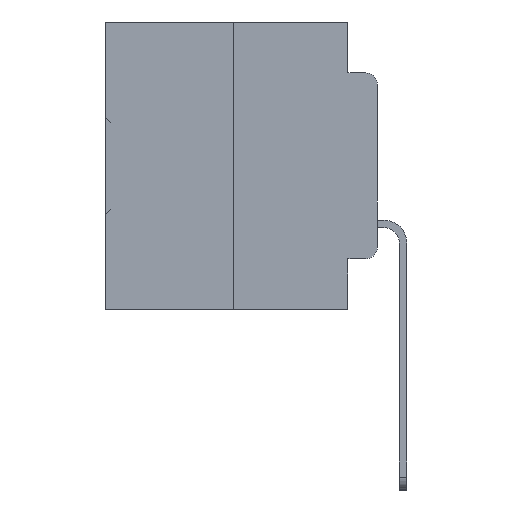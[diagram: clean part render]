
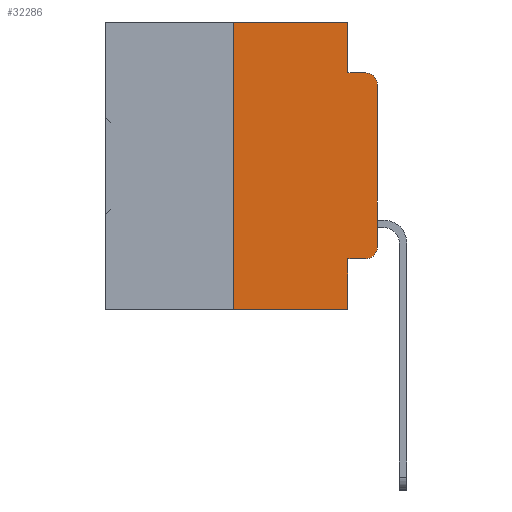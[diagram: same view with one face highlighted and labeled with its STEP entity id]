
A CAD part, left-side view. The second image highlights one B-rep face of the part: STEP entity #32286.
In plain terms, the highlighted planar face has unit normal (-1, 0, 0).
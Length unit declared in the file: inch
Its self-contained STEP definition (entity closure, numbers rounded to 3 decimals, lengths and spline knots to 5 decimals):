
#32 = EDGE_CURVE ( 'NONE', #3070, #14172, #7735, .T. ) ;
#1850 = DIRECTION ( 'NONE',  ( 0., 0., -1. ) ) ;
#1936 = VERTEX_POINT ( 'NONE', #9172 ) ;
#2328 = EDGE_CURVE ( 'NONE', #14172, #29148, #20751, .T. ) ;
#2523 = ORIENTED_EDGE ( 'NONE', *, *, #2328, .T. ) ;
#2650 = ORIENTED_EDGE ( 'NONE', *, *, #19686, .T. ) ;
#3070 = VERTEX_POINT ( 'NONE', #14114 ) ;
#3313 = ORIENTED_EDGE ( 'NONE', *, *, #5236, .F. ) ;
#3793 = CIRCLE ( 'NONE', #24096, 0.02 ) ;
#3899 = ORIENTED_EDGE ( 'NONE', *, *, #9823, .F. ) ;
#4029 = CARTESIAN_POINT ( 'NONE',  ( 0., 0.051, -0.0885 ) ) ;
#4086 = ORIENTED_EDGE ( 'NONE', *, *, #6081, .F. ) ;
#4285 = ORIENTED_EDGE ( 'NONE', *, *, #34201, .F. ) ;
#5115 = CARTESIAN_POINT ( 'NONE',  ( 0., 0.051, 0. ) ) ;
#5236 = EDGE_CURVE ( 'NONE', #16485, #1936, #21415, .T. ) ;
#5287 = ORIENTED_EDGE ( 'NONE', *, *, #8079, .T. ) ;
#5360 = ORIENTED_EDGE ( 'NONE', *, *, #6774, .F. ) ;
#5570 = CARTESIAN_POINT ( 'NONE',  ( 0., 0.25, 0. ) ) ;
#5973 = CARTESIAN_POINT ( 'NONE',  ( 0., 0.051, -0.0885 ) ) ;
#6081 = EDGE_CURVE ( 'NONE', #24636, #24177, #11952, .T. ) ;
#6456 = CARTESIAN_POINT ( 'NONE',  ( 0., 0.473, -0.5 ) ) ;
#6774 = EDGE_CURVE ( 'NONE', #10427, #34752, #24679, .T. ) ;
#6993 = ORIENTED_EDGE ( 'NONE', *, *, #25337, .T. ) ;
#7388 = PLANE ( 'NONE',  #17544 ) ;
#7418 = ORIENTED_EDGE ( 'NONE', *, *, #32, .T. ) ;
#7715 = VECTOR ( 'NONE', #22508, 39.37008 ) ;
#7735 = CIRCLE ( 'NONE', #28140, 0.02 ) ;
#8079 = EDGE_CURVE ( 'NONE', #11602, #34752, #12018, .T. ) ;
#9172 = CARTESIAN_POINT ( 'NONE',  ( 0., 0.02, -0.0885 ) ) ;
#9292 = VECTOR ( 'NONE', #30020, 39.37008 ) ;
#9823 = EDGE_CURVE ( 'NONE', #24177, #16485, #28070, .T. ) ;
#10196 = DIRECTION ( 'NONE',  ( 1., 0., 0. ) ) ;
#10427 = VERTEX_POINT ( 'NONE', #29548 ) ;
#11602 = VERTEX_POINT ( 'NONE', #20110 ) ;
#11652 = DIRECTION ( 'NONE',  ( 0., 0., 1. ) ) ;
#11952 = LINE ( 'NONE', #12339, #25570 ) ;
#12018 = LINE ( 'NONE', #6456, #20133 ) ;
#12339 = CARTESIAN_POINT ( 'NONE',  ( 0., 0.473, 0. ) ) ;
#12803 = CARTESIAN_POINT ( 'NONE',  ( 0., 0.051, -0.4115 ) ) ;
#13549 = VECTOR ( 'NONE', #11652, 39.37008 ) ;
#14114 = CARTESIAN_POINT ( 'NONE',  ( 0., 0.02, -0.4115 ) ) ;
#14172 = VERTEX_POINT ( 'NONE', #30657 ) ;
#15082 = DIRECTION ( 'NONE',  ( 0., -1., 0. ) ) ;
#15665 = DIRECTION ( 'NONE',  ( 0., -1., 0. ) ) ;
#16280 = DIRECTION ( 'NONE',  ( 0., 0., -1. ) ) ;
#16485 = VERTEX_POINT ( 'NONE', #4029 ) ;
#17544 = AXIS2_PLACEMENT_3D ( 'NONE', #18353, #10196, #29260 ) ;
#18353 = CARTESIAN_POINT ( 'NONE',  ( 0., 0.473, 0. ) ) ;
#18394 = FACE_OUTER_BOUND ( 'NONE', #20306, .T. ) ;
#18772 = CARTESIAN_POINT ( 'NONE',  ( 0., 0.25, 0. ) ) ;
#18903 = DIRECTION ( 'NONE',  ( -1., 0., 0. ) ) ;
#19545 = DIRECTION ( 'NONE',  ( 0., 0., 1. ) ) ;
#19686 = EDGE_CURVE ( 'NONE', #29148, #1936, #3793, .T. ) ;
#20110 = CARTESIAN_POINT ( 'NONE',  ( 0., 0.25, -0.5 ) ) ;
#20133 = VECTOR ( 'NONE', #25652, 39.37008 ) ;
#20306 = EDGE_LOOP ( 'NONE', ( #2523, #2650, #3313, #3899, #4086, #4285, #5287, #5360, #6993, #7418 ) ) ;
#20751 = LINE ( 'NONE', #22505, #13549 ) ;
#20830 = VECTOR ( 'NONE', #16280, 39.37008 ) ;
#21102 = VECTOR ( 'NONE', #15665, 39.37008 ) ;
#21415 = LINE ( 'NONE', #5973, #7715 ) ;
#22348 = CARTESIAN_POINT ( 'NONE',  ( 0., 0.051, 0. ) ) ;
#22498 = VECTOR ( 'NONE', #19545, 39.37008 ) ;
#22505 = CARTESIAN_POINT ( 'NONE',  ( 0., 0., 0. ) ) ;
#22508 = DIRECTION ( 'NONE',  ( 0., -1., 0. ) ) ;
#24096 = AXIS2_PLACEMENT_3D ( 'NONE', #35130, #18903, #1850 ) ;
#24177 = VERTEX_POINT ( 'NONE', #22348 ) ;
#24554 = CARTESIAN_POINT ( 'NONE',  ( 0., 0.051, 0. ) ) ;
#24636 = VERTEX_POINT ( 'NONE', #18772 ) ;
#24679 = LINE ( 'NONE', #24554, #9292 ) ;
#25337 = EDGE_CURVE ( 'NONE', #10427, #3070, #28322, .T. ) ;
#25570 = VECTOR ( 'NONE', #15082, 39.37008 ) ;
#25652 = DIRECTION ( 'NONE',  ( 0., -1., 0. ) ) ;
#25662 = CARTESIAN_POINT ( 'NONE',  ( 0., 0.051, -0.5 ) ) ;
#28070 = LINE ( 'NONE', #5115, #20830 ) ;
#28140 = AXIS2_PLACEMENT_3D ( 'NONE', #31738, #31607, #35825 ) ;
#28322 = LINE ( 'NONE', #12803, #21102 ) ;
#28586 = CARTESIAN_POINT ( 'NONE',  ( 0., 0., -0.1085 ) ) ;
#29148 = VERTEX_POINT ( 'NONE', #28586 ) ;
#29260 = DIRECTION ( 'NONE',  ( 0., 0., -1. ) ) ;
#29548 = CARTESIAN_POINT ( 'NONE',  ( 0., 0.051, -0.4115 ) ) ;
#30020 = DIRECTION ( 'NONE',  ( 0., 0., -1. ) ) ;
#30579 = LINE ( 'NONE', #5570, #22498 ) ;
#30657 = CARTESIAN_POINT ( 'NONE',  ( 0., 0., -0.3915 ) ) ;
#31607 = DIRECTION ( 'NONE',  ( -1., 0., 0. ) ) ;
#31738 = CARTESIAN_POINT ( 'NONE',  ( 0., 0.02, -0.3915 ) ) ;
#32286 = ADVANCED_FACE ( 'NONE', ( #18394 ), #7388, .F. ) ;
#34201 = EDGE_CURVE ( 'NONE', #11602, #24636, #30579, .T. ) ;
#34752 = VERTEX_POINT ( 'NONE', #25662 ) ;
#35130 = CARTESIAN_POINT ( 'NONE',  ( 0., 0.02, -0.1085 ) ) ;
#35825 = DIRECTION ( 'NONE',  ( 0., 0., -1. ) ) ;
